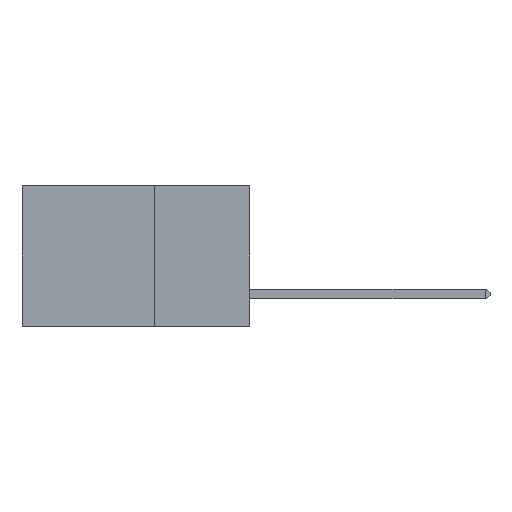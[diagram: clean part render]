
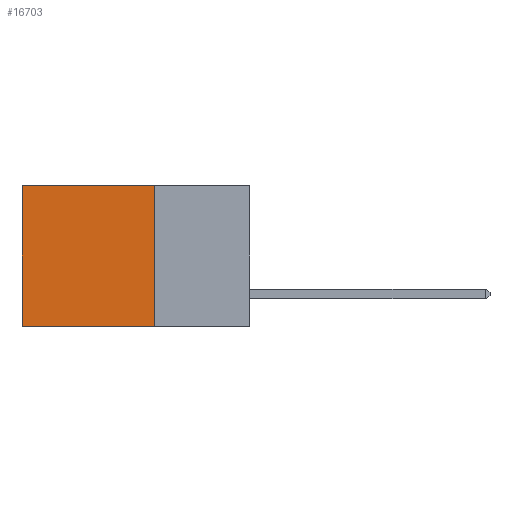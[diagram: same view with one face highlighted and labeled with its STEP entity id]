
A CAD part, left-side view. The second image highlights one B-rep face of the part: STEP entity #16703.
In plain terms, the highlighted planar face has unit normal (-1, 0, 0).
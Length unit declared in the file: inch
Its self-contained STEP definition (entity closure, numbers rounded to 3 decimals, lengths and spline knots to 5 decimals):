
#341 = LINE ( 'NONE', #685, #13602 ) ;
#685 = CARTESIAN_POINT ( 'NONE',  ( 0.2875, 0.25, -0.37 ) ) ;
#956 = AXIS2_PLACEMENT_3D ( 'NONE', #14406, #6737, #15680 ) ;
#1970 = LINE ( 'NONE', #6680, #5357 ) ;
#2540 = EDGE_CURVE ( 'NONE', #13404, #14157, #1970, .T. ) ;
#2597 = EDGE_LOOP ( 'NONE', ( #3948, #16379, #14138, #14810 ) ) ;
#3948 = ORIENTED_EDGE ( 'NONE', *, *, #13654, .T. ) ;
#5212 = CARTESIAN_POINT ( 'NONE',  ( 0.2875, 0.6, 0. ) ) ;
#5337 = EDGE_CURVE ( 'NONE', #14157, #6613, #341, .T. ) ;
#5357 = VECTOR ( 'NONE', #16891, 39.37008 ) ;
#5407 = PLANE ( 'NONE',  #956 ) ;
#6489 = DIRECTION ( 'NONE',  ( 0., 1., 0. ) ) ;
#6613 = VERTEX_POINT ( 'NONE', #13925 ) ;
#6680 = CARTESIAN_POINT ( 'NONE',  ( 0.2875, 0.25, 0. ) ) ;
#6737 = DIRECTION ( 'NONE',  ( 1., 0., 0. ) ) ;
#7176 = LINE ( 'NONE', #14923, #11011 ) ;
#7288 = DIRECTION ( 'NONE',  ( 0., 1., 0. ) ) ;
#11011 = VECTOR ( 'NONE', #16117, 39.37008 ) ;
#11762 = CARTESIAN_POINT ( 'NONE',  ( 0.2875, 0.25, 0. ) ) ;
#11857 = LINE ( 'NONE', #14933, #15578 ) ;
#12082 = VERTEX_POINT ( 'NONE', #5212 ) ;
#13073 = EDGE_CURVE ( 'NONE', #13404, #12082, #11857, .T. ) ;
#13404 = VERTEX_POINT ( 'NONE', #11762 ) ;
#13602 = VECTOR ( 'NONE', #6489, 39.37008 ) ;
#13654 = EDGE_CURVE ( 'NONE', #12082, #6613, #7176, .T. ) ;
#13925 = CARTESIAN_POINT ( 'NONE',  ( 0.2875, 0.6, -0.37 ) ) ;
#14138 = ORIENTED_EDGE ( 'NONE', *, *, #2540, .F. ) ;
#14157 = VERTEX_POINT ( 'NONE', #15997 ) ;
#14406 = CARTESIAN_POINT ( 'NONE',  ( 0.2875, 0.25, 0. ) ) ;
#14655 = FACE_OUTER_BOUND ( 'NONE', #2597, .T. ) ;
#14810 = ORIENTED_EDGE ( 'NONE', *, *, #13073, .T. ) ;
#14923 = CARTESIAN_POINT ( 'NONE',  ( 0.2875, 0.6, 0. ) ) ;
#14933 = CARTESIAN_POINT ( 'NONE',  ( 0.2875, 0.25, 0. ) ) ;
#15578 = VECTOR ( 'NONE', #7288, 39.37008 ) ;
#15680 = DIRECTION ( 'NONE',  ( 0., 0., -1. ) ) ;
#15997 = CARTESIAN_POINT ( 'NONE',  ( 0.2875, 0.25, -0.37 ) ) ;
#16117 = DIRECTION ( 'NONE',  ( 0., 0., -1. ) ) ;
#16379 = ORIENTED_EDGE ( 'NONE', *, *, #5337, .F. ) ;
#16703 = ADVANCED_FACE ( 'NONE', ( #14655 ), #5407, .F. ) ;
#16891 = DIRECTION ( 'NONE',  ( 0., 0., -1. ) ) ;
